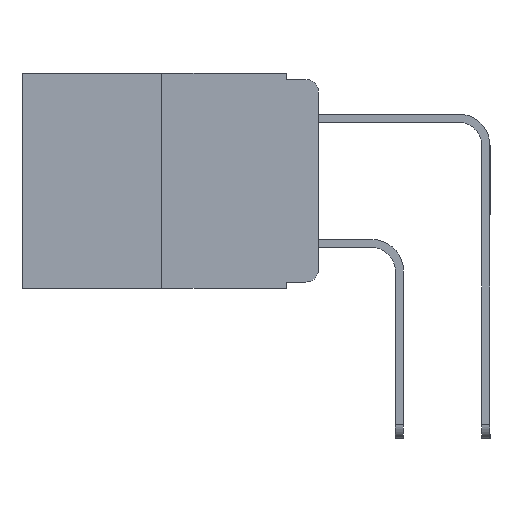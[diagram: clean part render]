
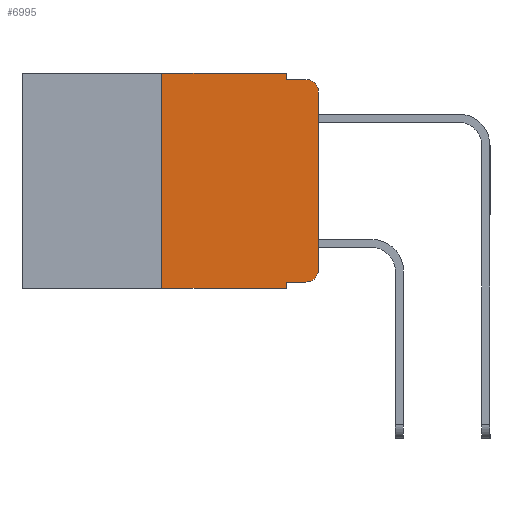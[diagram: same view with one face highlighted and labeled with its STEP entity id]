
A CAD part, left-side view. The second image highlights one B-rep face of the part: STEP entity #6995.
In plain terms, the highlighted planar face has unit normal (-1, 0, 0).
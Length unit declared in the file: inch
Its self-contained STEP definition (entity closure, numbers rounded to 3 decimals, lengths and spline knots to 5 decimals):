
#495 = DIRECTION ( 'NONE',  ( -1., 0., 0. ) ) ;
#654 = CIRCLE ( 'NONE', #2648, 0.02 ) ;
#901 = CARTESIAN_POINT ( 'NONE',  ( 0., 0., -0.313 ) ) ;
#1047 = LINE ( 'NONE', #22453, #5320 ) ;
#1238 = VERTEX_POINT ( 'NONE', #15745 ) ;
#2369 = EDGE_CURVE ( 'NONE', #6415, #16114, #19890, .T. ) ;
#2410 = DIRECTION ( 'NONE',  ( 0., 0., -1. ) ) ;
#2648 = AXIS2_PLACEMENT_3D ( 'NONE', #17114, #6226, #18925 ) ;
#2666 = CARTESIAN_POINT ( 'NONE',  ( 0., 0.051, -0.01 ) ) ;
#2964 = ORIENTED_EDGE ( 'NONE', *, *, #9685, .F. ) ;
#3537 = CARTESIAN_POINT ( 'NONE',  ( 0., 0.051, 0. ) ) ;
#3576 = LINE ( 'NONE', #9677, #22271 ) ;
#3645 = CARTESIAN_POINT ( 'NONE',  ( 0., 0.25, 0. ) ) ;
#4340 = EDGE_CURVE ( 'NONE', #23430, #21817, #9946, .T. ) ;
#5200 = CARTESIAN_POINT ( 'NONE',  ( 0., 0.25, -0.343 ) ) ;
#5320 = VECTOR ( 'NONE', #9847, 39.37008 ) ;
#5348 = LINE ( 'NONE', #17598, #20396 ) ;
#5374 = CIRCLE ( 'NONE', #10395, 0.02 ) ;
#5378 = DIRECTION ( 'NONE',  ( 0., 0., -1. ) ) ;
#5417 = EDGE_CURVE ( 'NONE', #21016, #1238, #1047, .T. ) ;
#5421 = PLANE ( 'NONE',  #8234 ) ;
#5456 = LINE ( 'NONE', #3537, #14581 ) ;
#5523 = CARTESIAN_POINT ( 'NONE',  ( 0., 0.051, -0.333 ) ) ;
#5944 = CARTESIAN_POINT ( 'NONE',  ( 0., 0.02, -0.333 ) ) ;
#6090 = ORIENTED_EDGE ( 'NONE', *, *, #11708, .F. ) ;
#6226 = DIRECTION ( 'NONE',  ( -1., 0., 0. ) ) ;
#6415 = VERTEX_POINT ( 'NONE', #5523 ) ;
#6660 = VERTEX_POINT ( 'NONE', #2666 ) ;
#6695 = CARTESIAN_POINT ( 'NONE',  ( 0., 0.051, -0.333 ) ) ;
#6995 = ADVANCED_FACE ( 'NONE', ( #23040 ), #5421, .F. ) ;
#7212 = EDGE_CURVE ( 'NONE', #6415, #1238, #18578, .T. ) ;
#7229 = CARTESIAN_POINT ( 'NONE',  ( 0., 0.473, 0. ) ) ;
#7370 = VERTEX_POINT ( 'NONE', #19126 ) ;
#7802 = ORIENTED_EDGE ( 'NONE', *, *, #23394, .T. ) ;
#8234 = AXIS2_PLACEMENT_3D ( 'NONE', #7229, #19948, #9080 ) ;
#9080 = DIRECTION ( 'NONE',  ( 0., 0., -1. ) ) ;
#9644 = CARTESIAN_POINT ( 'NONE',  ( 0., 0.051, 0. ) ) ;
#9677 = CARTESIAN_POINT ( 'NONE',  ( 0., 0.051, -0.01 ) ) ;
#9685 = EDGE_CURVE ( 'NONE', #21016, #13763, #14257, .T. ) ;
#9847 = DIRECTION ( 'NONE',  ( 0., -1., 0. ) ) ;
#9946 = LINE ( 'NONE', #13854, #18996 ) ;
#10108 = ORIENTED_EDGE ( 'NONE', *, *, #5417, .T. ) ;
#10395 = AXIS2_PLACEMENT_3D ( 'NONE', #11444, #495, #13260 ) ;
#10581 = VECTOR ( 'NONE', #14554, 39.37008 ) ;
#11444 = CARTESIAN_POINT ( 'NONE',  ( 0., 0.02, -0.03 ) ) ;
#11708 = EDGE_CURVE ( 'NONE', #13763, #7370, #5348, .T. ) ;
#11801 = ORIENTED_EDGE ( 'NONE', *, *, #20600, .T. ) ;
#12315 = VERTEX_POINT ( 'NONE', #17817 ) ;
#13260 = DIRECTION ( 'NONE',  ( 0., 0., -1. ) ) ;
#13763 = VERTEX_POINT ( 'NONE', #21065 ) ;
#13768 = VECTOR ( 'NONE', #2410, 39.37008 ) ;
#13854 = CARTESIAN_POINT ( 'NONE',  ( 0., 0., 0. ) ) ;
#13967 = DIRECTION ( 'NONE',  ( 0., -1., 0. ) ) ;
#14257 = LINE ( 'NONE', #3645, #10581 ) ;
#14554 = DIRECTION ( 'NONE',  ( 0., 0., 1. ) ) ;
#14581 = VECTOR ( 'NONE', #5378, 39.37008 ) ;
#14640 = ORIENTED_EDGE ( 'NONE', *, *, #15746, .F. ) ;
#15226 = ORIENTED_EDGE ( 'NONE', *, *, #2369, .T. ) ;
#15668 = DIRECTION ( 'NONE',  ( 0., 0., 1. ) ) ;
#15745 = CARTESIAN_POINT ( 'NONE',  ( 0., 0.051, -0.343 ) ) ;
#15746 = EDGE_CURVE ( 'NONE', #7370, #6660, #5456, .T. ) ;
#16041 = EDGE_LOOP ( 'NONE', ( #18018, #11801, #17170, #14640, #6090, #2964, #10108, #21970, #15226, #7802 ) ) ;
#16114 = VERTEX_POINT ( 'NONE', #5944 ) ;
#17114 = CARTESIAN_POINT ( 'NONE',  ( 0., 0.02, -0.313 ) ) ;
#17170 = ORIENTED_EDGE ( 'NONE', *, *, #18190, .F. ) ;
#17598 = CARTESIAN_POINT ( 'NONE',  ( 0., 0.473, 0. ) ) ;
#17817 = CARTESIAN_POINT ( 'NONE',  ( 0., 0.02, -0.01 ) ) ;
#18018 = ORIENTED_EDGE ( 'NONE', *, *, #4340, .T. ) ;
#18190 = EDGE_CURVE ( 'NONE', #6660, #12315, #3576, .T. ) ;
#18578 = LINE ( 'NONE', #9644, #13768 ) ;
#18925 = DIRECTION ( 'NONE',  ( 0., 0., -1. ) ) ;
#18996 = VECTOR ( 'NONE', #15668, 39.37008 ) ;
#19126 = CARTESIAN_POINT ( 'NONE',  ( 0., 0.051, 0. ) ) ;
#19393 = DIRECTION ( 'NONE',  ( 0., -1., 0. ) ) ;
#19890 = LINE ( 'NONE', #6695, #20449 ) ;
#19948 = DIRECTION ( 'NONE',  ( 1., 0., 0. ) ) ;
#20166 = CARTESIAN_POINT ( 'NONE',  ( 0., 0., -0.03 ) ) ;
#20396 = VECTOR ( 'NONE', #19393, 39.37008 ) ;
#20449 = VECTOR ( 'NONE', #13967, 39.37008 ) ;
#20591 = DIRECTION ( 'NONE',  ( 0., -1., 0. ) ) ;
#20600 = EDGE_CURVE ( 'NONE', #21817, #12315, #5374, .T. ) ;
#21016 = VERTEX_POINT ( 'NONE', #5200 ) ;
#21065 = CARTESIAN_POINT ( 'NONE',  ( 0., 0.25, 0. ) ) ;
#21817 = VERTEX_POINT ( 'NONE', #20166 ) ;
#21970 = ORIENTED_EDGE ( 'NONE', *, *, #7212, .F. ) ;
#22271 = VECTOR ( 'NONE', #20591, 39.37008 ) ;
#22453 = CARTESIAN_POINT ( 'NONE',  ( 0., 0.473, -0.343 ) ) ;
#23040 = FACE_OUTER_BOUND ( 'NONE', #16041, .T. ) ;
#23394 = EDGE_CURVE ( 'NONE', #16114, #23430, #654, .T. ) ;
#23430 = VERTEX_POINT ( 'NONE', #901 ) ;
